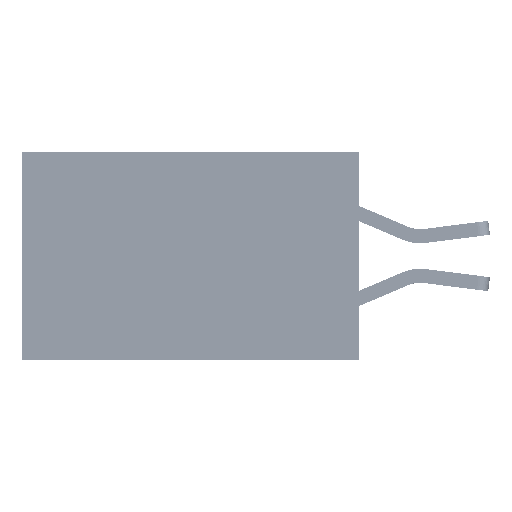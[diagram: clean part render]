
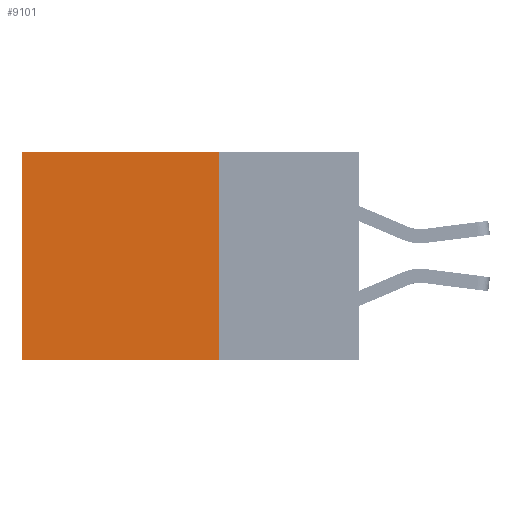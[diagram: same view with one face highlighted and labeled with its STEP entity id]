
A CAD part, left-side view. The second image highlights one B-rep face of the part: STEP entity #9101.
In plain terms, the highlighted planar face has unit normal (-1, 0, 0).
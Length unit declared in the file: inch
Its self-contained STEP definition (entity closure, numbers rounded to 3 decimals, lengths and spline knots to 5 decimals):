
#965 = CARTESIAN_POINT ( 'NONE',  ( 0.2875, 0.25, 0. ) ) ;
#1010 = CARTESIAN_POINT ( 'NONE',  ( 0.2875, 0.25, 0. ) ) ;
#1057 = VERTEX_POINT ( 'NONE', #24074 ) ;
#1382 = CARTESIAN_POINT ( 'NONE',  ( 0.2875, 0.25, -0.37 ) ) ;
#2111 = LINE ( 'NONE', #2585, #21025 ) ;
#2585 = CARTESIAN_POINT ( 'NONE',  ( 0.2875, 0.25, 0. ) ) ;
#3208 = CARTESIAN_POINT ( 'NONE',  ( 0.2875, 0.25, 0. ) ) ;
#4504 = DIRECTION ( 'NONE',  ( 0., 0., -1. ) ) ;
#7282 = DIRECTION ( 'NONE',  ( 1., 0., 0. ) ) ;
#7425 = EDGE_CURVE ( 'NONE', #9338, #30228, #2111, .T. ) ;
#8934 = LINE ( 'NONE', #1010, #36042 ) ;
#9101 = ADVANCED_FACE ( 'NONE', ( #43426 ), #18691, .F. ) ;
#9338 = VERTEX_POINT ( 'NONE', #3208 ) ;
#10598 = DIRECTION ( 'NONE',  ( 0., 0., -1. ) ) ;
#10791 = DIRECTION ( 'NONE',  ( 0., 0., -1. ) ) ;
#13091 = VERTEX_POINT ( 'NONE', #1382 ) ;
#13365 = CARTESIAN_POINT ( 'NONE',  ( 0.2875, 0.6, 0. ) ) ;
#14095 = LINE ( 'NONE', #36021, #28591 ) ;
#15593 = DIRECTION ( 'NONE',  ( 0., 1., 0. ) ) ;
#18691 = PLANE ( 'NONE',  #28596 ) ;
#21025 = VECTOR ( 'NONE', #23819, 39.37008 ) ;
#23819 = DIRECTION ( 'NONE',  ( 0., 1., 0. ) ) ;
#24018 = ORIENTED_EDGE ( 'NONE', *, *, #29761, .T. ) ;
#24074 = CARTESIAN_POINT ( 'NONE',  ( 0.2875, 0.6, -0.37 ) ) ;
#25875 = LINE ( 'NONE', #41008, #30919 ) ;
#28230 = ORIENTED_EDGE ( 'NONE', *, *, #29967, .F. ) ;
#28591 = VECTOR ( 'NONE', #10598, 39.37008 ) ;
#28596 = AXIS2_PLACEMENT_3D ( 'NONE', #965, #7282, #10791 ) ;
#29761 = EDGE_CURVE ( 'NONE', #30228, #1057, #14095, .T. ) ;
#29967 = EDGE_CURVE ( 'NONE', #9338, #13091, #8934, .T. ) ;
#30228 = VERTEX_POINT ( 'NONE', #13365 ) ;
#30919 = VECTOR ( 'NONE', #15593, 39.37008 ) ;
#36021 = CARTESIAN_POINT ( 'NONE',  ( 0.2875, 0.6, 0. ) ) ;
#36042 = VECTOR ( 'NONE', #4504, 39.37008 ) ;
#41008 = CARTESIAN_POINT ( 'NONE',  ( 0.2875, 0.25, -0.37 ) ) ;
#41650 = EDGE_CURVE ( 'NONE', #13091, #1057, #25875, .T. ) ;
#43426 = FACE_OUTER_BOUND ( 'NONE', #43711, .T. ) ;
#43711 = EDGE_LOOP ( 'NONE', ( #24018, #44512, #28230, #43742 ) ) ;
#43742 = ORIENTED_EDGE ( 'NONE', *, *, #7425, .T. ) ;
#44512 = ORIENTED_EDGE ( 'NONE', *, *, #41650, .F. ) ;
